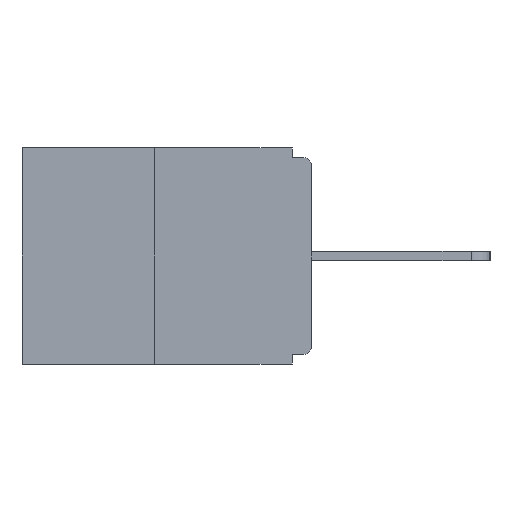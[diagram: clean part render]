
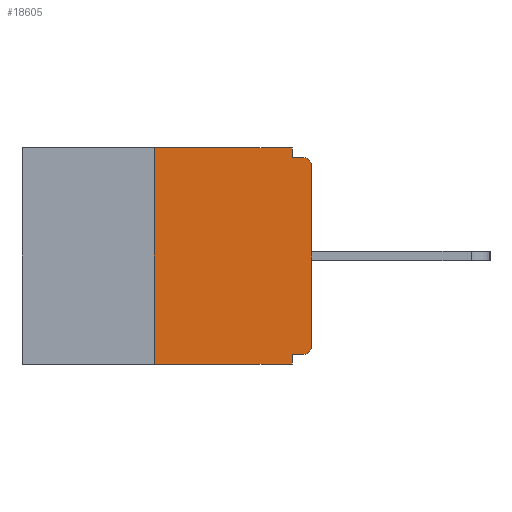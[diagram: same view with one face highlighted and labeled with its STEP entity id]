
A CAD part, left-side view. The second image highlights one B-rep face of the part: STEP entity #18605.
In plain terms, the highlighted planar face has unit normal (-1, 0, 0).
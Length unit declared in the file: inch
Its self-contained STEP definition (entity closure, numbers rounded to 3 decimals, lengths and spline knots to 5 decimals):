
#297 = VERTEX_POINT ( 'NONE', #1643 ) ;
#310 = CARTESIAN_POINT ( 'NONE',  ( 0., 0., -0.313 ) ) ;
#759 = VERTEX_POINT ( 'NONE', #14387 ) ;
#879 = CIRCLE ( 'NONE', #14967, 0.015 ) ;
#1003 = CARTESIAN_POINT ( 'NONE',  ( 0., 0.031, 0. ) ) ;
#1255 = DIRECTION ( 'NONE',  ( 0., 0., -1. ) ) ;
#1629 = CARTESIAN_POINT ( 'NONE',  ( 0., 0.015, -0.328 ) ) ;
#1636 = EDGE_CURVE ( 'NONE', #7884, #297, #10731, .T. ) ;
#1637 = CARTESIAN_POINT ( 'NONE',  ( 0., 0., -0.328 ) ) ;
#1643 = CARTESIAN_POINT ( 'NONE',  ( 0., 0.031, -0.343 ) ) ;
#1830 = AXIS2_PLACEMENT_3D ( 'NONE', #11691, #8824, #15979 ) ;
#1834 = LINE ( 'NONE', #11182, #16001 ) ;
#2539 = DIRECTION ( 'NONE',  ( 0., 0., 1. ) ) ;
#2753 = EDGE_CURVE ( 'NONE', #7871, #17591, #11118, .T. ) ;
#2822 = EDGE_CURVE ( 'NONE', #14262, #7884, #13007, .T. ) ;
#3019 = DIRECTION ( 'NONE',  ( 0., -1., 0. ) ) ;
#3032 = VECTOR ( 'NONE', #4412, 39.37008 ) ;
#3088 = DIRECTION ( 'NONE',  ( 0., 1., 0. ) ) ;
#3312 = CARTESIAN_POINT ( 'NONE',  ( 0., 0.25, -0.343 ) ) ;
#3386 = EDGE_LOOP ( 'NONE', ( #14115, #7865, #14719, #13877, #3956, #15354, #4638, #6236, #7886, #13452 ) ) ;
#3956 = ORIENTED_EDGE ( 'NONE', *, *, #2822, .F. ) ;
#4220 = LINE ( 'NONE', #16788, #8119 ) ;
#4412 = DIRECTION ( 'NONE',  ( 0., -1., 0. ) ) ;
#4638 = ORIENTED_EDGE ( 'NONE', *, *, #17244, .T. ) ;
#5117 = LINE ( 'NONE', #10301, #16317 ) ;
#5292 = AXIS2_PLACEMENT_3D ( 'NONE', #9890, #14315, #5475 ) ;
#5475 = DIRECTION ( 'NONE',  ( 0., 0., -1. ) ) ;
#5801 = VERTEX_POINT ( 'NONE', #3312 ) ;
#6065 = VERTEX_POINT ( 'NONE', #11930 ) ;
#6236 = ORIENTED_EDGE ( 'NONE', *, *, #15508, .T. ) ;
#6305 = EDGE_CURVE ( 'NONE', #5801, #297, #9692, .T. ) ;
#6990 = DIRECTION ( 'NONE',  ( -1., 0., 0. ) ) ;
#7214 = CARTESIAN_POINT ( 'NONE',  ( 0., 0.031, -0.343 ) ) ;
#7364 = CARTESIAN_POINT ( 'NONE',  ( 0., 0.46, -0.343 ) ) ;
#7396 = VECTOR ( 'NONE', #3019, 39.37008 ) ;
#7481 = PLANE ( 'NONE',  #1830 ) ;
#7491 = VECTOR ( 'NONE', #3088, 39.37008 ) ;
#7865 = ORIENTED_EDGE ( 'NONE', *, *, #9807, .F. ) ;
#7871 = VERTEX_POINT ( 'NONE', #10472 ) ;
#7884 = VERTEX_POINT ( 'NONE', #13493 ) ;
#7886 = ORIENTED_EDGE ( 'NONE', *, *, #17778, .F. ) ;
#8119 = VECTOR ( 'NONE', #18160, 39.37008 ) ;
#8475 = DIRECTION ( 'NONE',  ( 0., 0., -1. ) ) ;
#8706 = CIRCLE ( 'NONE', #5292, 0.015 ) ;
#8824 = DIRECTION ( 'NONE',  ( 1., 0., 0. ) ) ;
#8830 = VERTEX_POINT ( 'NONE', #310 ) ;
#9692 = LINE ( 'NONE', #7364, #7396 ) ;
#9807 = EDGE_CURVE ( 'NONE', #5801, #9942, #1834, .T. ) ;
#9890 = CARTESIAN_POINT ( 'NONE',  ( 0., 0.015, -0.03 ) ) ;
#9942 = VERTEX_POINT ( 'NONE', #11692 ) ;
#10248 = CARTESIAN_POINT ( 'NONE',  ( 0., 0.46, 0. ) ) ;
#10301 = CARTESIAN_POINT ( 'NONE',  ( 0., 0., -0.015 ) ) ;
#10467 = VECTOR ( 'NONE', #1255, 39.37008 ) ;
#10472 = CARTESIAN_POINT ( 'NONE',  ( 0., 0.031, 0. ) ) ;
#10731 = LINE ( 'NONE', #7214, #15769 ) ;
#11118 = LINE ( 'NONE', #1003, #10467 ) ;
#11182 = CARTESIAN_POINT ( 'NONE',  ( 0., 0.25, 0. ) ) ;
#11378 = EDGE_CURVE ( 'NONE', #14262, #8830, #879, .T. ) ;
#11489 = FACE_OUTER_BOUND ( 'NONE', #3386, .T. ) ;
#11691 = CARTESIAN_POINT ( 'NONE',  ( 0., 0.46, 0. ) ) ;
#11692 = CARTESIAN_POINT ( 'NONE',  ( 0., 0.25, 0. ) ) ;
#11930 = CARTESIAN_POINT ( 'NONE',  ( 0., 0., -0.03 ) ) ;
#13007 = LINE ( 'NONE', #1637, #7491 ) ;
#13452 = ORIENTED_EDGE ( 'NONE', *, *, #2753, .F. ) ;
#13493 = CARTESIAN_POINT ( 'NONE',  ( 0., 0.031, -0.328 ) ) ;
#13877 = ORIENTED_EDGE ( 'NONE', *, *, #1636, .F. ) ;
#14115 = ORIENTED_EDGE ( 'NONE', *, *, #14164, .F. ) ;
#14164 = EDGE_CURVE ( 'NONE', #9942, #7871, #17612, .T. ) ;
#14262 = VERTEX_POINT ( 'NONE', #1629 ) ;
#14315 = DIRECTION ( 'NONE',  ( -1., 0., 0. ) ) ;
#14387 = CARTESIAN_POINT ( 'NONE',  ( 0., 0.015, -0.015 ) ) ;
#14719 = ORIENTED_EDGE ( 'NONE', *, *, #6305, .T. ) ;
#14967 = AXIS2_PLACEMENT_3D ( 'NONE', #15753, #6990, #8475 ) ;
#15354 = ORIENTED_EDGE ( 'NONE', *, *, #11378, .T. ) ;
#15508 = EDGE_CURVE ( 'NONE', #6065, #759, #8706, .T. ) ;
#15675 = CARTESIAN_POINT ( 'NONE',  ( 0., 0.031, -0.015 ) ) ;
#15753 = CARTESIAN_POINT ( 'NONE',  ( 0., 0.015, -0.313 ) ) ;
#15769 = VECTOR ( 'NONE', #17273, 39.37008 ) ;
#15979 = DIRECTION ( 'NONE',  ( 0., 0., -1. ) ) ;
#16001 = VECTOR ( 'NONE', #2539, 39.37008 ) ;
#16036 = DIRECTION ( 'NONE',  ( 0., -1., 0. ) ) ;
#16317 = VECTOR ( 'NONE', #16036, 39.37008 ) ;
#16788 = CARTESIAN_POINT ( 'NONE',  ( 0., 0., 0. ) ) ;
#17244 = EDGE_CURVE ( 'NONE', #8830, #6065, #4220, .T. ) ;
#17273 = DIRECTION ( 'NONE',  ( 0., 0., -1. ) ) ;
#17591 = VERTEX_POINT ( 'NONE', #15675 ) ;
#17612 = LINE ( 'NONE', #10248, #3032 ) ;
#17778 = EDGE_CURVE ( 'NONE', #17591, #759, #5117, .T. ) ;
#18160 = DIRECTION ( 'NONE',  ( 0., 0., 1. ) ) ;
#18605 = ADVANCED_FACE ( 'NONE', ( #11489 ), #7481, .F. ) ;
